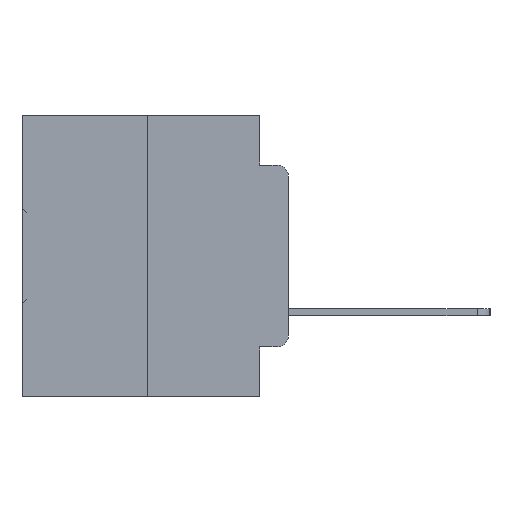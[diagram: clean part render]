
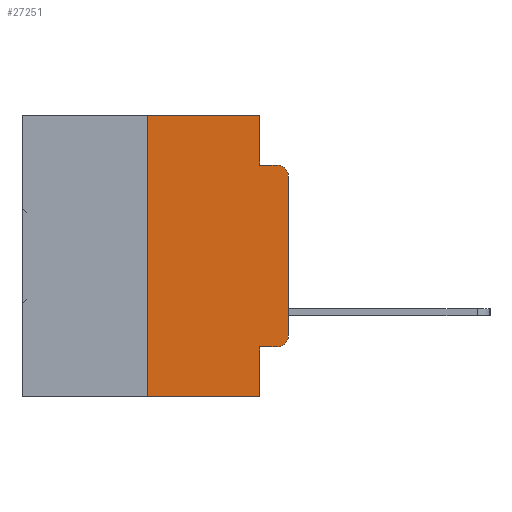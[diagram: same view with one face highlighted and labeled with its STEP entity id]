
A CAD part, left-side view. The second image highlights one B-rep face of the part: STEP entity #27251.
In plain terms, the highlighted planar face has unit normal (-1, 0, 0).
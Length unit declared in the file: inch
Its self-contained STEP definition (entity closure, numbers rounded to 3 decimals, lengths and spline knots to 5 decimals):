
#1083 = VECTOR ( 'NONE', #13055, 39.37008 ) ;
#1796 = LINE ( 'NONE', #24395, #29024 ) ;
#2334 = VECTOR ( 'NONE', #7314, 39.37008 ) ;
#2374 = EDGE_CURVE ( 'NONE', #13093, #31508, #33937, .T. ) ;
#3040 = EDGE_CURVE ( 'NONE', #16041, #23521, #32368, .T. ) ;
#3109 = AXIS2_PLACEMENT_3D ( 'NONE', #4504, #23070, #7166 ) ;
#4504 = CARTESIAN_POINT ( 'NONE',  ( 0., 0.02, -0.1085 ) ) ;
#4810 = VERTEX_POINT ( 'NONE', #4993 ) ;
#4993 = CARTESIAN_POINT ( 'NONE',  ( 0., 0.051, -0.0885 ) ) ;
#5535 = PLANE ( 'NONE',  #33943 ) ;
#5887 = ORIENTED_EDGE ( 'NONE', *, *, #2374, .T. ) ;
#7042 = CARTESIAN_POINT ( 'NONE',  ( 0., 0.25, 0. ) ) ;
#7159 = CARTESIAN_POINT ( 'NONE',  ( 0., 0.051, 0. ) ) ;
#7166 = DIRECTION ( 'NONE',  ( 0., 0., -1. ) ) ;
#7314 = DIRECTION ( 'NONE',  ( 0., -1., 0. ) ) ;
#7667 = ORIENTED_EDGE ( 'NONE', *, *, #25838, .T. ) ;
#7672 = DIRECTION ( 'NONE',  ( 0., 0., 1. ) ) ;
#8190 = DIRECTION ( 'NONE',  ( 1., 0., 0. ) ) ;
#8414 = EDGE_CURVE ( 'NONE', #27304, #4810, #19786, .T. ) ;
#8462 = ORIENTED_EDGE ( 'NONE', *, *, #19276, .F. ) ;
#8507 = FACE_OUTER_BOUND ( 'NONE', #12826, .T. ) ;
#9039 = CARTESIAN_POINT ( 'NONE',  ( 0., 0.02, -0.3915 ) ) ;
#9785 = DIRECTION ( 'NONE',  ( 0., -1., 0. ) ) ;
#9940 = VERTEX_POINT ( 'NONE', #19089 ) ;
#10230 = EDGE_CURVE ( 'NONE', #4810, #9940, #22709, .T. ) ;
#11757 = DIRECTION ( 'NONE',  ( 0., 0., -1. ) ) ;
#12416 = VECTOR ( 'NONE', #7672, 39.37008 ) ;
#12770 = CARTESIAN_POINT ( 'NONE',  ( 0., 0., -0.1085 ) ) ;
#12826 = EDGE_LOOP ( 'NONE', ( #5887, #20020, #33356, #21331, #28185, #22982, #13124, #8462, #13153, #7667 ) ) ;
#13055 = DIRECTION ( 'NONE',  ( 0., -1., 0. ) ) ;
#13093 = VERTEX_POINT ( 'NONE', #15619 ) ;
#13124 = ORIENTED_EDGE ( 'NONE', *, *, #26142, .T. ) ;
#13153 = ORIENTED_EDGE ( 'NONE', *, *, #28638, .T. ) ;
#13293 = CIRCLE ( 'NONE', #3109, 0.02 ) ;
#15243 = DIRECTION ( 'NONE',  ( 0., 0., -1. ) ) ;
#15619 = CARTESIAN_POINT ( 'NONE',  ( 0., 0., -0.3915 ) ) ;
#16041 = VERTEX_POINT ( 'NONE', #18829 ) ;
#16487 = DIRECTION ( 'NONE',  ( 0., -1., 0. ) ) ;
#17323 = VECTOR ( 'NONE', #33377, 39.37008 ) ;
#17363 = EDGE_CURVE ( 'NONE', #31508, #9940, #13293, .T. ) ;
#18829 = CARTESIAN_POINT ( 'NONE',  ( 0., 0.25, -0.5 ) ) ;
#19073 = CARTESIAN_POINT ( 'NONE',  ( 0., 0.25, 0. ) ) ;
#19089 = CARTESIAN_POINT ( 'NONE',  ( 0., 0.02, -0.0885 ) ) ;
#19231 = VECTOR ( 'NONE', #9785, 39.37008 ) ;
#19276 = EDGE_CURVE ( 'NONE', #30173, #21546, #25073, .T. ) ;
#19786 = LINE ( 'NONE', #7159, #32665 ) ;
#20020 = ORIENTED_EDGE ( 'NONE', *, *, #17363, .T. ) ;
#20042 = CARTESIAN_POINT ( 'NONE',  ( 0., 0.051, -0.5 ) ) ;
#20662 = CARTESIAN_POINT ( 'NONE',  ( 0., 0.051, -0.4115 ) ) ;
#21331 = ORIENTED_EDGE ( 'NONE', *, *, #8414, .F. ) ;
#21546 = VERTEX_POINT ( 'NONE', #20042 ) ;
#21729 = DIRECTION ( 'NONE',  ( 0., 0., 1. ) ) ;
#22709 = LINE ( 'NONE', #23228, #2334 ) ;
#22806 = EDGE_CURVE ( 'NONE', #23521, #27304, #26181, .T. ) ;
#22982 = ORIENTED_EDGE ( 'NONE', *, *, #3040, .F. ) ;
#23070 = DIRECTION ( 'NONE',  ( -1., 0., 0. ) ) ;
#23228 = CARTESIAN_POINT ( 'NONE',  ( 0., 0.051, -0.0885 ) ) ;
#23521 = VERTEX_POINT ( 'NONE', #7042 ) ;
#24047 = CARTESIAN_POINT ( 'NONE',  ( 0., 0.473, 0. ) ) ;
#24341 = CIRCLE ( 'NONE', #24500, 0.02 ) ;
#24395 = CARTESIAN_POINT ( 'NONE',  ( 0., 0.051, -0.4115 ) ) ;
#24500 = AXIS2_PLACEMENT_3D ( 'NONE', #9039, #27437, #11757 ) ;
#25073 = LINE ( 'NONE', #28268, #17323 ) ;
#25838 = EDGE_CURVE ( 'NONE', #26227, #13093, #24341, .T. ) ;
#26142 = EDGE_CURVE ( 'NONE', #16041, #21546, #28330, .T. ) ;
#26181 = LINE ( 'NONE', #28018, #19231 ) ;
#26227 = VERTEX_POINT ( 'NONE', #26307 ) ;
#26307 = CARTESIAN_POINT ( 'NONE',  ( 0., 0.02, -0.4115 ) ) ;
#26622 = DIRECTION ( 'NONE',  ( 0., 0., -1. ) ) ;
#27251 = ADVANCED_FACE ( 'NONE', ( #8507 ), #5535, .F. ) ;
#27304 = VERTEX_POINT ( 'NONE', #31858 ) ;
#27437 = DIRECTION ( 'NONE',  ( -1., 0., 0. ) ) ;
#28018 = CARTESIAN_POINT ( 'NONE',  ( 0., 0.473, 0. ) ) ;
#28185 = ORIENTED_EDGE ( 'NONE', *, *, #22806, .F. ) ;
#28268 = CARTESIAN_POINT ( 'NONE',  ( 0., 0.051, 0. ) ) ;
#28330 = LINE ( 'NONE', #28670, #1083 ) ;
#28638 = EDGE_CURVE ( 'NONE', #30173, #26227, #1796, .T. ) ;
#28670 = CARTESIAN_POINT ( 'NONE',  ( 0., 0.473, -0.5 ) ) ;
#29024 = VECTOR ( 'NONE', #16487, 39.37008 ) ;
#30173 = VERTEX_POINT ( 'NONE', #20662 ) ;
#31508 = VERTEX_POINT ( 'NONE', #12770 ) ;
#31595 = VECTOR ( 'NONE', #21729, 39.37008 ) ;
#31858 = CARTESIAN_POINT ( 'NONE',  ( 0., 0.051, 0. ) ) ;
#32368 = LINE ( 'NONE', #19073, #31595 ) ;
#32665 = VECTOR ( 'NONE', #15243, 39.37008 ) ;
#33356 = ORIENTED_EDGE ( 'NONE', *, *, #10230, .F. ) ;
#33377 = DIRECTION ( 'NONE',  ( 0., 0., -1. ) ) ;
#33718 = CARTESIAN_POINT ( 'NONE',  ( 0., 0., 0. ) ) ;
#33937 = LINE ( 'NONE', #33718, #12416 ) ;
#33943 = AXIS2_PLACEMENT_3D ( 'NONE', #24047, #8190, #26622 ) ;
